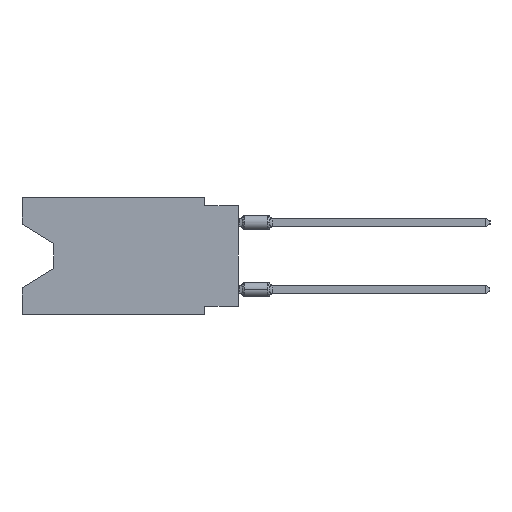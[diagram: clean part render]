
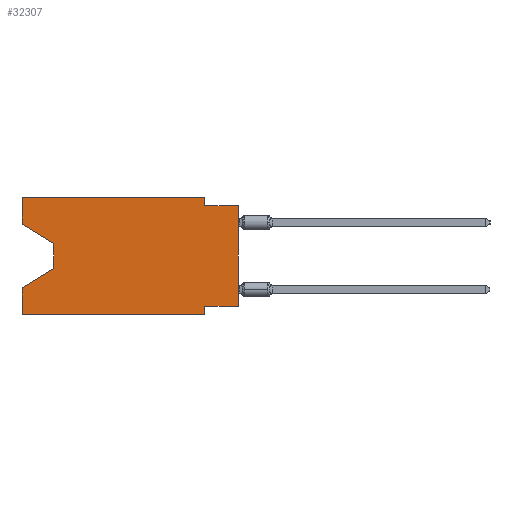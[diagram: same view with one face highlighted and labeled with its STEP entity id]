
A CAD part, left-side view. The second image highlights one B-rep face of the part: STEP entity #32307.
In plain terms, the highlighted planar face has unit normal (-1, 0, 0).
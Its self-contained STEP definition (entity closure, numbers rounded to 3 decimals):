
#1260 = CARTESIAN_POINT ( 'NONE',  ( 0., 16.383, -8.89 ) ) ;
#1686 = CARTESIAN_POINT ( 'NONE',  ( 0., 0., -0.635 ) ) ;
#1849 = VERTEX_POINT ( 'NONE', #7611 ) ;
#1910 = DIRECTION ( 'NONE',  ( 0., 0.855, -0.519 ) ) ;
#3539 = ORIENTED_EDGE ( 'NONE', *, *, #53422, .T. ) ;
#4226 = DIRECTION ( 'NONE',  ( 0., -0.855, -0.519 ) ) ;
#5121 = LINE ( 'NONE', #55681, #27212 ) ;
#5306 = ORIENTED_EDGE ( 'NONE', *, *, #39208, .T. ) ;
#5509 = CARTESIAN_POINT ( 'NONE',  ( 0., 2.54, -8.255 ) ) ;
#5752 = DIRECTION ( 'NONE',  ( 0., -1., 0. ) ) ;
#5793 = LINE ( 'NONE', #21095, #60301 ) ;
#6877 = VERTEX_POINT ( 'NONE', #29597 ) ;
#7611 = CARTESIAN_POINT ( 'NONE',  ( 0., 2.54, -8.89 ) ) ;
#8138 = VERTEX_POINT ( 'NONE', #46292 ) ;
#8169 = ORIENTED_EDGE ( 'NONE', *, *, #23164, .F. ) ;
#8986 = EDGE_CURVE ( 'NONE', #16686, #62518, #40802, .T. ) ;
#9044 = VERTEX_POINT ( 'NONE', #58064 ) ;
#11189 = DIRECTION ( 'NONE',  ( 0., -1., 0. ) ) ;
#12276 = PLANE ( 'NONE',  #44409 ) ;
#12942 = ORIENTED_EDGE ( 'NONE', *, *, #33798, .F. ) ;
#13711 = ORIENTED_EDGE ( 'NONE', *, *, #65254, .T. ) ;
#13916 = EDGE_CURVE ( 'NONE', #35546, #37704, #42421, .T. ) ;
#13933 = LINE ( 'NONE', #34208, #24727 ) ;
#15692 = EDGE_LOOP ( 'NONE', ( #3539, #13711, #5306, #44555, #25302, #18905, #12942, #56143, #8169, #25720, #22840, #30759 ) ) ;
#15894 = DIRECTION ( 'NONE',  ( 0., 1., 0. ) ) ;
#16553 = CARTESIAN_POINT ( 'NONE',  ( 0., 2.54, 0. ) ) ;
#16686 = VERTEX_POINT ( 'NONE', #39047 ) ;
#17063 = VECTOR ( 'NONE', #47762, 1000. ) ;
#17263 = CARTESIAN_POINT ( 'NONE',  ( 0., 16.383, 0. ) ) ;
#18548 = VECTOR ( 'NONE', #60067, 1000. ) ;
#18905 = ORIENTED_EDGE ( 'NONE', *, *, #57933, .F. ) ;
#20092 = DIRECTION ( 'NONE',  ( 0., 0., 1. ) ) ;
#21095 = CARTESIAN_POINT ( 'NONE',  ( 0., 16.383, 0. ) ) ;
#21386 = CARTESIAN_POINT ( 'NONE',  ( 0., 16.383, -8.89 ) ) ;
#21639 = EDGE_CURVE ( 'NONE', #25893, #36240, #5121, .T. ) ;
#21827 = CARTESIAN_POINT ( 'NONE',  ( 0., 16.383, 0. ) ) ;
#21962 = DIRECTION ( 'NONE',  ( 0., -1., 0. ) ) ;
#22824 = CARTESIAN_POINT ( 'NONE',  ( 0., 13.97, -5.385 ) ) ;
#22840 = ORIENTED_EDGE ( 'NONE', *, *, #8986, .F. ) ;
#23164 = EDGE_CURVE ( 'NONE', #36880, #36240, #52240, .T. ) ;
#24727 = VECTOR ( 'NONE', #51184, 1000. ) ;
#25302 = ORIENTED_EDGE ( 'NONE', *, *, #35927, .T. ) ;
#25720 = ORIENTED_EDGE ( 'NONE', *, *, #28172, .F. ) ;
#25893 = VERTEX_POINT ( 'NONE', #33789 ) ;
#26080 = DIRECTION ( 'NONE',  ( 0., 0., 1. ) ) ;
#27184 = LINE ( 'NONE', #16553, #37614 ) ;
#27212 = VECTOR ( 'NONE', #20092, 1000. ) ;
#28172 = EDGE_CURVE ( 'NONE', #62518, #36880, #27184, .T. ) ;
#29597 = CARTESIAN_POINT ( 'NONE',  ( 0., 13.97, -5.385 ) ) ;
#30759 = ORIENTED_EDGE ( 'NONE', *, *, #61990, .F. ) ;
#32307 = ADVANCED_FACE ( 'NONE', ( #62534 ), #12276, .F. ) ;
#33789 = CARTESIAN_POINT ( 'NONE',  ( 0., 0., -8.255 ) ) ;
#33798 = EDGE_CURVE ( 'NONE', #25893, #57893, #61154, .T. ) ;
#34208 = CARTESIAN_POINT ( 'NONE',  ( 0., 13.97, -3.505 ) ) ;
#35546 = VERTEX_POINT ( 'NONE', #1260 ) ;
#35736 = CARTESIAN_POINT ( 'NONE',  ( 0., 2.54, -0.635 ) ) ;
#35927 = EDGE_CURVE ( 'NONE', #35546, #1849, #51320, .T. ) ;
#36240 = VERTEX_POINT ( 'NONE', #54470 ) ;
#36880 = VERTEX_POINT ( 'NONE', #35736 ) ;
#37413 = CARTESIAN_POINT ( 'NONE',  ( 0., 16.383, 0. ) ) ;
#37543 = DIRECTION ( 'NONE',  ( 0., 0., -1. ) ) ;
#37614 = VECTOR ( 'NONE', #47485, 1000. ) ;
#37704 = VERTEX_POINT ( 'NONE', #37783 ) ;
#37783 = CARTESIAN_POINT ( 'NONE',  ( 0., 16.383, -6.852 ) ) ;
#37809 = VECTOR ( 'NONE', #4226, 1000. ) ;
#38484 = CARTESIAN_POINT ( 'NONE',  ( 0., 2.54, 0. ) ) ;
#39047 = CARTESIAN_POINT ( 'NONE',  ( 0., 16.383, 0. ) ) ;
#39208 = EDGE_CURVE ( 'NONE', #6877, #37704, #47463, .T. ) ;
#40802 = LINE ( 'NONE', #21827, #57437 ) ;
#42400 = VECTOR ( 'NONE', #15894, 1000. ) ;
#42421 = LINE ( 'NONE', #37413, #17063 ) ;
#44145 = LINE ( 'NONE', #49810, #37809 ) ;
#44409 = AXIS2_PLACEMENT_3D ( 'NONE', #17263, #62212, #37543 ) ;
#44555 = ORIENTED_EDGE ( 'NONE', *, *, #13916, .F. ) ;
#44878 = CARTESIAN_POINT ( 'NONE',  ( 0., 0., -8.255 ) ) ;
#46292 = CARTESIAN_POINT ( 'NONE',  ( 0., 16.383, -2.038 ) ) ;
#47463 = LINE ( 'NONE', #22824, #59916 ) ;
#47485 = DIRECTION ( 'NONE',  ( 0., 0., -1. ) ) ;
#47762 = DIRECTION ( 'NONE',  ( 0., 0., 1. ) ) ;
#49810 = CARTESIAN_POINT ( 'NONE',  ( 0., 16.383, -2.038 ) ) ;
#51184 = DIRECTION ( 'NONE',  ( 0., 0., -1. ) ) ;
#51320 = LINE ( 'NONE', #21386, #57333 ) ;
#52240 = LINE ( 'NONE', #1686, #58291 ) ;
#53422 = EDGE_CURVE ( 'NONE', #8138, #9044, #44145, .T. ) ;
#54470 = CARTESIAN_POINT ( 'NONE',  ( 0., 0., -0.635 ) ) ;
#55681 = CARTESIAN_POINT ( 'NONE',  ( 0., 0., 0. ) ) ;
#56073 = CARTESIAN_POINT ( 'NONE',  ( 0., 2.54, -8.89 ) ) ;
#56143 = ORIENTED_EDGE ( 'NONE', *, *, #21639, .T. ) ;
#57333 = VECTOR ( 'NONE', #5752, 1000. ) ;
#57437 = VECTOR ( 'NONE', #11189, 1000. ) ;
#57893 = VERTEX_POINT ( 'NONE', #5509 ) ;
#57933 = EDGE_CURVE ( 'NONE', #57893, #1849, #61058, .T. ) ;
#58064 = CARTESIAN_POINT ( 'NONE',  ( 0., 13.97, -3.505 ) ) ;
#58291 = VECTOR ( 'NONE', #21962, 1000. ) ;
#59916 = VECTOR ( 'NONE', #1910, 1000. ) ;
#60067 = DIRECTION ( 'NONE',  ( 0., 0., -1. ) ) ;
#60301 = VECTOR ( 'NONE', #26080, 1000. ) ;
#61058 = LINE ( 'NONE', #56073, #18548 ) ;
#61154 = LINE ( 'NONE', #44878, #42400 ) ;
#61990 = EDGE_CURVE ( 'NONE', #8138, #16686, #5793, .T. ) ;
#62212 = DIRECTION ( 'NONE',  ( 1., 0., 0. ) ) ;
#62518 = VERTEX_POINT ( 'NONE', #38484 ) ;
#62534 = FACE_OUTER_BOUND ( 'NONE', #15692, .T. ) ;
#65254 = EDGE_CURVE ( 'NONE', #9044, #6877, #13933, .T. ) ;
